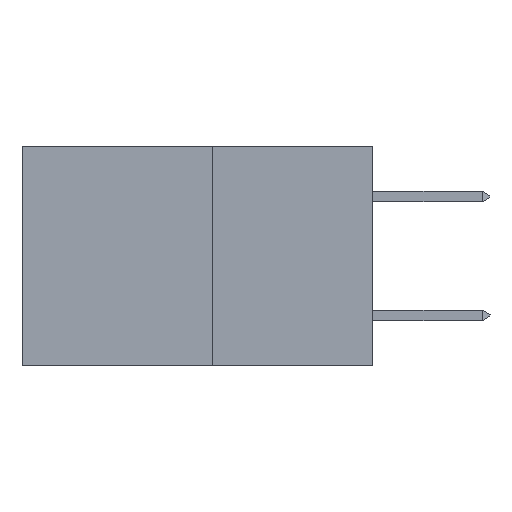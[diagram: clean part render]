
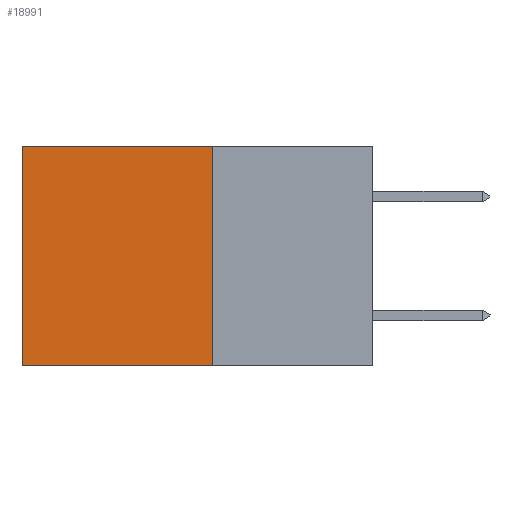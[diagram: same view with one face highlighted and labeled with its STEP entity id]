
A CAD part, left-side view. The second image highlights one B-rep face of the part: STEP entity #18991.
In plain terms, the highlighted planar face has unit normal (-1, 0, 0).
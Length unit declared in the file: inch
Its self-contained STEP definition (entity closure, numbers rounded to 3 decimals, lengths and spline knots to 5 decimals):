
#460 = CARTESIAN_POINT ( 'NONE',  ( 0.277, 0.59, -0.37 ) ) ;
#1093 = LINE ( 'NONE', #9994, #12902 ) ;
#1748 = VERTEX_POINT ( 'NONE', #13261 ) ;
#2026 = LINE ( 'NONE', #12974, #11705 ) ;
#2772 = CARTESIAN_POINT ( 'NONE',  ( 0.277, 0.27, -0.37 ) ) ;
#2988 = CARTESIAN_POINT ( 'NONE',  ( 0.277, 0.59, 0. ) ) ;
#3000 = ORIENTED_EDGE ( 'NONE', *, *, #10958, .F. ) ;
#3487 = ORIENTED_EDGE ( 'NONE', *, *, #18795, .T. ) ;
#3733 = DIRECTION ( 'NONE',  ( 0., 1., 0. ) ) ;
#4520 = ORIENTED_EDGE ( 'NONE', *, *, #14555, .T. ) ;
#4564 = EDGE_CURVE ( 'NONE', #18599, #18675, #16147, .T. ) ;
#4979 = CARTESIAN_POINT ( 'NONE',  ( 0.277, 0.27, -0.37 ) ) ;
#7285 = EDGE_LOOP ( 'NONE', ( #3487, #14023, #3000, #4520 ) ) ;
#7317 = LINE ( 'NONE', #8006, #18914 ) ;
#7872 = DIRECTION ( 'NONE',  ( 0., 0., -1. ) ) ;
#8006 = CARTESIAN_POINT ( 'NONE',  ( 0.277, 0.27, -0.37 ) ) ;
#8916 = CARTESIAN_POINT ( 'NONE',  ( 0.277, 0.27, -0.37 ) ) ;
#9994 = CARTESIAN_POINT ( 'NONE',  ( 0.277, 0.59, -0.37 ) ) ;
#10447 = DIRECTION ( 'NONE',  ( 0., 0., -1. ) ) ;
#10958 = EDGE_CURVE ( 'NONE', #1748, #18599, #7317, .T. ) ;
#11705 = VECTOR ( 'NONE', #3733, 39.37008 ) ;
#12902 = VECTOR ( 'NONE', #16047, 39.37008 ) ;
#12943 = VERTEX_POINT ( 'NONE', #2988 ) ;
#12974 = CARTESIAN_POINT ( 'NONE',  ( 0.277, 0.27, 0. ) ) ;
#13261 = CARTESIAN_POINT ( 'NONE',  ( 0.277, 0.27, 0. ) ) ;
#13620 = FACE_OUTER_BOUND ( 'NONE', #7285, .T. ) ;
#14023 = ORIENTED_EDGE ( 'NONE', *, *, #4564, .F. ) ;
#14477 = DIRECTION ( 'NONE',  ( 0., 1., 0. ) ) ;
#14555 = EDGE_CURVE ( 'NONE', #1748, #12943, #2026, .T. ) ;
#15661 = VECTOR ( 'NONE', #14477, 39.37008 ) ;
#16047 = DIRECTION ( 'NONE',  ( 0., 0., -1. ) ) ;
#16147 = LINE ( 'NONE', #2772, #15661 ) ;
#18023 = PLANE ( 'NONE',  #18034 ) ;
#18034 = AXIS2_PLACEMENT_3D ( 'NONE', #8916, #19543, #10447 ) ;
#18599 = VERTEX_POINT ( 'NONE', #4979 ) ;
#18675 = VERTEX_POINT ( 'NONE', #460 ) ;
#18795 = EDGE_CURVE ( 'NONE', #12943, #18675, #1093, .T. ) ;
#18914 = VECTOR ( 'NONE', #7872, 39.37008 ) ;
#18991 = ADVANCED_FACE ( 'NONE', ( #13620 ), #18023, .F. ) ;
#19543 = DIRECTION ( 'NONE',  ( 1., 0., 0. ) ) ;
